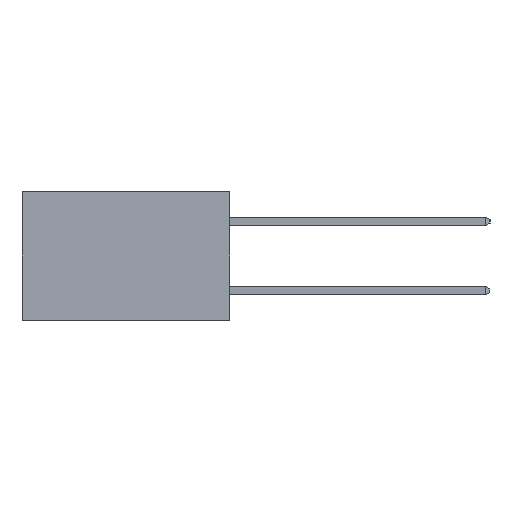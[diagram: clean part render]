
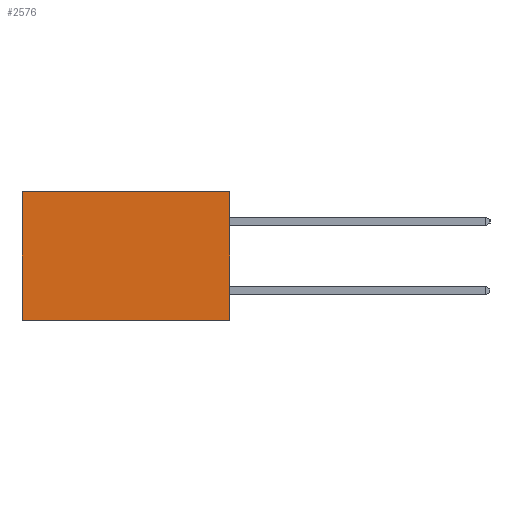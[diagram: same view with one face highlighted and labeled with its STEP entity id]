
A CAD part, left-side view. The second image highlights one B-rep face of the part: STEP entity #2576.
In plain terms, the highlighted planar face has unit normal (-1, 0, 0).
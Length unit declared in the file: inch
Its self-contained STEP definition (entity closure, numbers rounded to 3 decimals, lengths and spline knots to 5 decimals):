
#952 = AXIS2_PLACEMENT_3D ( 'NONE', #14384, #16487, #12238 ) ;
#2056 = LINE ( 'NONE', #10746, #2505 ) ;
#2064 = CARTESIAN_POINT ( 'NONE',  ( 0.298, 0., -0.37 ) ) ;
#2324 = CARTESIAN_POINT ( 'NONE',  ( 0.298, 0., 0. ) ) ;
#2505 = VECTOR ( 'NONE', #4211, 39.37008 ) ;
#2576 = ADVANCED_FACE ( 'NONE', ( #8562 ), #7066, .F. ) ;
#2983 = VERTEX_POINT ( 'NONE', #13215 ) ;
#3396 = DIRECTION ( 'NONE',  ( 0., 1., 0. ) ) ;
#3636 = DIRECTION ( 'NONE',  ( 0., 0., -1. ) ) ;
#3695 = CARTESIAN_POINT ( 'NONE',  ( 0.298, 0.6, 0. ) ) ;
#3714 = CARTESIAN_POINT ( 'NONE',  ( 0.298, 0.6, -0.37 ) ) ;
#4211 = DIRECTION ( 'NONE',  ( 0., 0., -1. ) ) ;
#4420 = ORIENTED_EDGE ( 'NONE', *, *, #16659, .T. ) ;
#4542 = LINE ( 'NONE', #2064, #14544 ) ;
#5432 = CARTESIAN_POINT ( 'NONE',  ( 0.298, 0., 0. ) ) ;
#5826 = CARTESIAN_POINT ( 'NONE',  ( 0.298, 0., 0. ) ) ;
#7066 = PLANE ( 'NONE',  #952 ) ;
#7083 = VERTEX_POINT ( 'NONE', #5432 ) ;
#7301 = EDGE_LOOP ( 'NONE', ( #11769, #9509, #14623, #4420 ) ) ;
#7657 = EDGE_CURVE ( 'NONE', #9401, #14547, #2056, .T. ) ;
#7938 = EDGE_CURVE ( 'NONE', #2983, #14547, #4542, .T. ) ;
#8562 = FACE_OUTER_BOUND ( 'NONE', #7301, .T. ) ;
#9375 = EDGE_CURVE ( 'NONE', #7083, #2983, #10211, .T. ) ;
#9401 = VERTEX_POINT ( 'NONE', #3695 ) ;
#9509 = ORIENTED_EDGE ( 'NONE', *, *, #7938, .F. ) ;
#10211 = LINE ( 'NONE', #2324, #16573 ) ;
#10746 = CARTESIAN_POINT ( 'NONE',  ( 0.298, 0.6, 0. ) ) ;
#11769 = ORIENTED_EDGE ( 'NONE', *, *, #7657, .T. ) ;
#12238 = DIRECTION ( 'NONE',  ( 0., 0., -1. ) ) ;
#12322 = VECTOR ( 'NONE', #14989, 39.37008 ) ;
#13215 = CARTESIAN_POINT ( 'NONE',  ( 0.298, 0., -0.37 ) ) ;
#14384 = CARTESIAN_POINT ( 'NONE',  ( 0.298, 0., 0. ) ) ;
#14544 = VECTOR ( 'NONE', #3396, 39.37008 ) ;
#14547 = VERTEX_POINT ( 'NONE', #3714 ) ;
#14623 = ORIENTED_EDGE ( 'NONE', *, *, #9375, .F. ) ;
#14989 = DIRECTION ( 'NONE',  ( 0., 1., 0. ) ) ;
#15716 = LINE ( 'NONE', #5826, #12322 ) ;
#16487 = DIRECTION ( 'NONE',  ( 1., 0., 0. ) ) ;
#16573 = VECTOR ( 'NONE', #3636, 39.37008 ) ;
#16659 = EDGE_CURVE ( 'NONE', #7083, #9401, #15716, .T. ) ;
